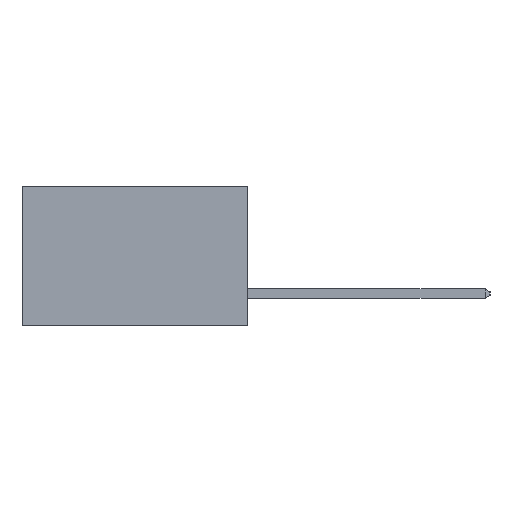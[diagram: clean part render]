
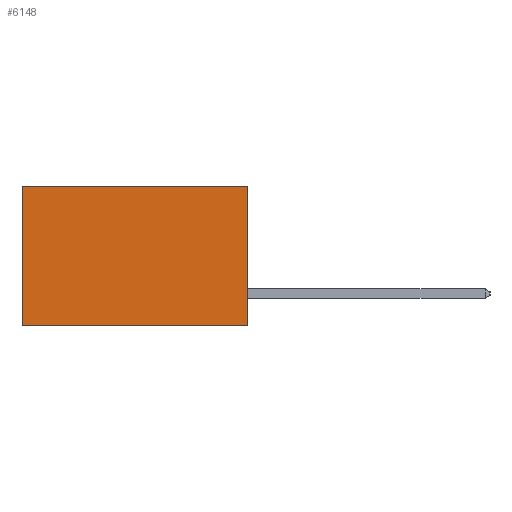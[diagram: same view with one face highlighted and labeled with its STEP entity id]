
A CAD part, left-side view. The second image highlights one B-rep face of the part: STEP entity #6148.
In plain terms, the highlighted planar face has unit normal (-1, 0, 0).
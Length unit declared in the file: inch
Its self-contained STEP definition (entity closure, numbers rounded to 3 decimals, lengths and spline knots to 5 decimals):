
#448 = CARTESIAN_POINT ( 'NONE',  ( 0.298, 0., 0. ) ) ;
#976 = DIRECTION ( 'NONE',  ( 0., 1., 0. ) ) ;
#1434 = EDGE_CURVE ( 'NONE', #13964, #4629, #10921, .T. ) ;
#2045 = DIRECTION ( 'NONE',  ( 0., 0., -1. ) ) ;
#2751 = PLANE ( 'NONE',  #13418 ) ;
#2950 = CARTESIAN_POINT ( 'NONE',  ( 0.298, 0., -0.37 ) ) ;
#3249 = EDGE_CURVE ( 'NONE', #13964, #7944, #18680, .T. ) ;
#3272 = CARTESIAN_POINT ( 'NONE',  ( 0.298, 0.6, 0. ) ) ;
#4629 = VERTEX_POINT ( 'NONE', #3272 ) ;
#4888 = CARTESIAN_POINT ( 'NONE',  ( 0.298, 0., 0. ) ) ;
#6079 = CARTESIAN_POINT ( 'NONE',  ( 0.298, 0., 0. ) ) ;
#6148 = ADVANCED_FACE ( 'NONE', ( #10741 ), #2751, .F. ) ;
#6474 = EDGE_CURVE ( 'NONE', #7944, #13714, #12707, .T. ) ;
#7106 = CARTESIAN_POINT ( 'NONE',  ( 0.298, 0., 0. ) ) ;
#7455 = CARTESIAN_POINT ( 'NONE',  ( 0.298, 0., -0.37 ) ) ;
#7620 = DIRECTION ( 'NONE',  ( 0., 1., 0. ) ) ;
#7944 = VERTEX_POINT ( 'NONE', #2950 ) ;
#7996 = DIRECTION ( 'NONE',  ( 0., 0., -1. ) ) ;
#8226 = EDGE_CURVE ( 'NONE', #4629, #13714, #14250, .T. ) ;
#9241 = EDGE_LOOP ( 'NONE', ( #9937, #18888, #15147, #14613 ) ) ;
#9937 = ORIENTED_EDGE ( 'NONE', *, *, #8226, .T. ) ;
#10381 = VECTOR ( 'NONE', #976, 39.37008 ) ;
#10610 = VECTOR ( 'NONE', #18761, 39.37008 ) ;
#10623 = VECTOR ( 'NONE', #2045, 39.37008 ) ;
#10741 = FACE_OUTER_BOUND ( 'NONE', #9241, .T. ) ;
#10921 = LINE ( 'NONE', #448, #10381 ) ;
#12707 = LINE ( 'NONE', #7455, #16177 ) ;
#13400 = CARTESIAN_POINT ( 'NONE',  ( 0.298, 0.6, 0. ) ) ;
#13418 = AXIS2_PLACEMENT_3D ( 'NONE', #6079, #16255, #7996 ) ;
#13714 = VERTEX_POINT ( 'NONE', #15402 ) ;
#13964 = VERTEX_POINT ( 'NONE', #4888 ) ;
#14250 = LINE ( 'NONE', #13400, #10623 ) ;
#14613 = ORIENTED_EDGE ( 'NONE', *, *, #1434, .T. ) ;
#15147 = ORIENTED_EDGE ( 'NONE', *, *, #3249, .F. ) ;
#15402 = CARTESIAN_POINT ( 'NONE',  ( 0.298, 0.6, -0.37 ) ) ;
#16177 = VECTOR ( 'NONE', #7620, 39.37008 ) ;
#16255 = DIRECTION ( 'NONE',  ( 1., 0., 0. ) ) ;
#18680 = LINE ( 'NONE', #7106, #10610 ) ;
#18761 = DIRECTION ( 'NONE',  ( 0., 0., -1. ) ) ;
#18888 = ORIENTED_EDGE ( 'NONE', *, *, #6474, .F. ) ;
